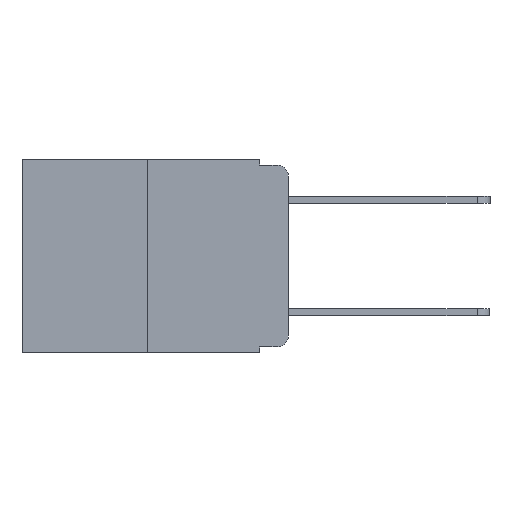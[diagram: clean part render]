
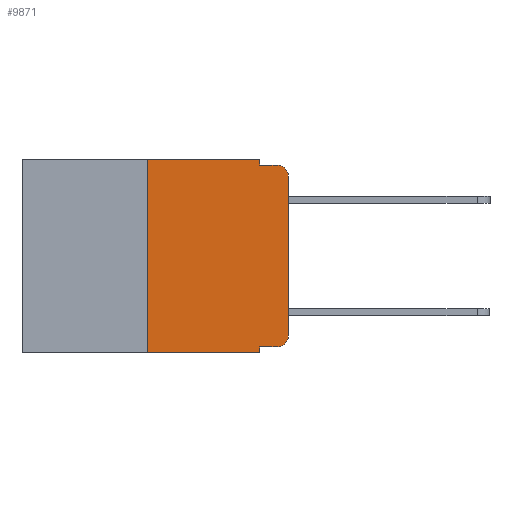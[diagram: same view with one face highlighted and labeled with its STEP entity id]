
A CAD part, left-side view. The second image highlights one B-rep face of the part: STEP entity #9871.
In plain terms, the highlighted planar face has unit normal (-1, 0, 0).
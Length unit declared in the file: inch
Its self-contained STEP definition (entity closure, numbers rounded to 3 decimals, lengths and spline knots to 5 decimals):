
#246 = CARTESIAN_POINT ( 'NONE',  ( 0., 0., -0.03 ) ) ;
#722 = DIRECTION ( 'NONE',  ( 0., 0., 1. ) ) ;
#753 = EDGE_LOOP ( 'NONE', ( #6237, #3652, #13315, #10500, #12760, #3201, #4537, #2432, #15533, #15996 ) ) ;
#1021 = VERTEX_POINT ( 'NONE', #3219 ) ;
#1023 = VERTEX_POINT ( 'NONE', #13635 ) ;
#1217 = CARTESIAN_POINT ( 'NONE',  ( 0., 0.051, 0. ) ) ;
#1225 = LINE ( 'NONE', #7362, #8525 ) ;
#1258 = VERTEX_POINT ( 'NONE', #246 ) ;
#2209 = LINE ( 'NONE', #2960, #9873 ) ;
#2432 = ORIENTED_EDGE ( 'NONE', *, *, #12095, .F. ) ;
#2960 = CARTESIAN_POINT ( 'NONE',  ( 0., 0.25, 0. ) ) ;
#3201 = ORIENTED_EDGE ( 'NONE', *, *, #12024, .F. ) ;
#3219 = CARTESIAN_POINT ( 'NONE',  ( 0., 0.02, -0.01 ) ) ;
#3395 = VERTEX_POINT ( 'NONE', #4117 ) ;
#3652 = ORIENTED_EDGE ( 'NONE', *, *, #11840, .T. ) ;
#3835 = VECTOR ( 'NONE', #8543, 39.37008 ) ;
#4117 = CARTESIAN_POINT ( 'NONE',  ( 0., 0.25, -0.343 ) ) ;
#4537 = ORIENTED_EDGE ( 'NONE', *, *, #10649, .T. ) ;
#4666 = VERTEX_POINT ( 'NONE', #8051 ) ;
#4722 = LINE ( 'NONE', #9919, #14358 ) ;
#4881 = DIRECTION ( 'NONE',  ( 1., 0., 0. ) ) ;
#5585 = CARTESIAN_POINT ( 'NONE',  ( 0., 0.473, 0. ) ) ;
#5841 = FACE_OUTER_BOUND ( 'NONE', #753, .T. ) ;
#6006 = LINE ( 'NONE', #10175, #15031 ) ;
#6064 = AXIS2_PLACEMENT_3D ( 'NONE', #9175, #4881, #14090 ) ;
#6164 = CARTESIAN_POINT ( 'NONE',  ( 0., 0.02, -0.313 ) ) ;
#6237 = ORIENTED_EDGE ( 'NONE', *, *, #11804, .T. ) ;
#6668 = DIRECTION ( 'NONE',  ( -1., 0., 0. ) ) ;
#6897 = VERTEX_POINT ( 'NONE', #10050 ) ;
#6937 = CIRCLE ( 'NONE', #9985, 0.02 ) ;
#7309 = AXIS2_PLACEMENT_3D ( 'NONE', #6164, #15102, #7630 ) ;
#7362 = CARTESIAN_POINT ( 'NONE',  ( 0., 0.051, -0.333 ) ) ;
#7630 = DIRECTION ( 'NONE',  ( 0., 0., -1. ) ) ;
#7633 = CARTESIAN_POINT ( 'NONE',  ( 0., 0.473, -0.343 ) ) ;
#7693 = PLANE ( 'NONE',  #6064 ) ;
#7866 = VERTEX_POINT ( 'NONE', #16356 ) ;
#8042 = CARTESIAN_POINT ( 'NONE',  ( 0., 0., 0. ) ) ;
#8051 = CARTESIAN_POINT ( 'NONE',  ( 0., 0.25, 0. ) ) ;
#8086 = LINE ( 'NONE', #1217, #3835 ) ;
#8485 = DIRECTION ( 'NONE',  ( 0., -1., 0. ) ) ;
#8525 = VECTOR ( 'NONE', #8850, 39.37008 ) ;
#8543 = DIRECTION ( 'NONE',  ( 0., 0., -1. ) ) ;
#8850 = DIRECTION ( 'NONE',  ( 0., -1., 0. ) ) ;
#8909 = EDGE_CURVE ( 'NONE', #4666, #1023, #9964, .T. ) ;
#9032 = VERTEX_POINT ( 'NONE', #16125 ) ;
#9175 = CARTESIAN_POINT ( 'NONE',  ( 0., 0.473, 0. ) ) ;
#9871 = ADVANCED_FACE ( 'NONE', ( #5841 ), #7693, .F. ) ;
#9873 = VECTOR ( 'NONE', #12536, 39.37008 ) ;
#9919 = CARTESIAN_POINT ( 'NONE',  ( 0., 0.051, -0.01 ) ) ;
#9964 = LINE ( 'NONE', #5585, #15440 ) ;
#9985 = AXIS2_PLACEMENT_3D ( 'NONE', #14397, #6668, #15475 ) ;
#10050 = CARTESIAN_POINT ( 'NONE',  ( 0., 0.051, -0.01 ) ) ;
#10065 = CARTESIAN_POINT ( 'NONE',  ( 0., 0.051, -0.333 ) ) ;
#10175 = CARTESIAN_POINT ( 'NONE',  ( 0., 0.051, 0. ) ) ;
#10500 = ORIENTED_EDGE ( 'NONE', *, *, #11974, .F. ) ;
#10649 = EDGE_CURVE ( 'NONE', #3395, #9032, #11829, .T. ) ;
#11053 = VECTOR ( 'NONE', #16158, 39.37008 ) ;
#11234 = CARTESIAN_POINT ( 'NONE',  ( 0., 0., -0.313 ) ) ;
#11804 = EDGE_CURVE ( 'NONE', #12855, #1258, #11815, .T. ) ;
#11815 = LINE ( 'NONE', #8042, #16667 ) ;
#11829 = LINE ( 'NONE', #7633, #11053 ) ;
#11840 = EDGE_CURVE ( 'NONE', #1258, #1021, #6937, .T. ) ;
#11970 = EDGE_CURVE ( 'NONE', #6897, #1021, #4722, .T. ) ;
#11974 = EDGE_CURVE ( 'NONE', #1023, #6897, #8086, .T. ) ;
#11992 = CIRCLE ( 'NONE', #7309, 0.02 ) ;
#12024 = EDGE_CURVE ( 'NONE', #3395, #4666, #2209, .T. ) ;
#12095 = EDGE_CURVE ( 'NONE', #16971, #9032, #6006, .T. ) ;
#12096 = EDGE_CURVE ( 'NONE', #16971, #7866, #1225, .T. ) ;
#12171 = EDGE_CURVE ( 'NONE', #7866, #12855, #11992, .T. ) ;
#12536 = DIRECTION ( 'NONE',  ( 0., 0., 1. ) ) ;
#12760 = ORIENTED_EDGE ( 'NONE', *, *, #8909, .F. ) ;
#12855 = VERTEX_POINT ( 'NONE', #11234 ) ;
#13315 = ORIENTED_EDGE ( 'NONE', *, *, #11970, .F. ) ;
#13635 = CARTESIAN_POINT ( 'NONE',  ( 0., 0.051, 0. ) ) ;
#13801 = DIRECTION ( 'NONE',  ( 0., 0., -1. ) ) ;
#14090 = DIRECTION ( 'NONE',  ( 0., 0., -1. ) ) ;
#14358 = VECTOR ( 'NONE', #8485, 39.37008 ) ;
#14397 = CARTESIAN_POINT ( 'NONE',  ( 0., 0.02, -0.03 ) ) ;
#14615 = DIRECTION ( 'NONE',  ( 0., -1., 0. ) ) ;
#15031 = VECTOR ( 'NONE', #13801, 39.37008 ) ;
#15102 = DIRECTION ( 'NONE',  ( -1., 0., 0. ) ) ;
#15440 = VECTOR ( 'NONE', #14615, 39.37008 ) ;
#15475 = DIRECTION ( 'NONE',  ( 0., 0., -1. ) ) ;
#15533 = ORIENTED_EDGE ( 'NONE', *, *, #12096, .T. ) ;
#15996 = ORIENTED_EDGE ( 'NONE', *, *, #12171, .T. ) ;
#16125 = CARTESIAN_POINT ( 'NONE',  ( 0., 0.051, -0.343 ) ) ;
#16158 = DIRECTION ( 'NONE',  ( 0., -1., 0. ) ) ;
#16356 = CARTESIAN_POINT ( 'NONE',  ( 0., 0.02, -0.333 ) ) ;
#16667 = VECTOR ( 'NONE', #722, 39.37008 ) ;
#16971 = VERTEX_POINT ( 'NONE', #10065 ) ;
